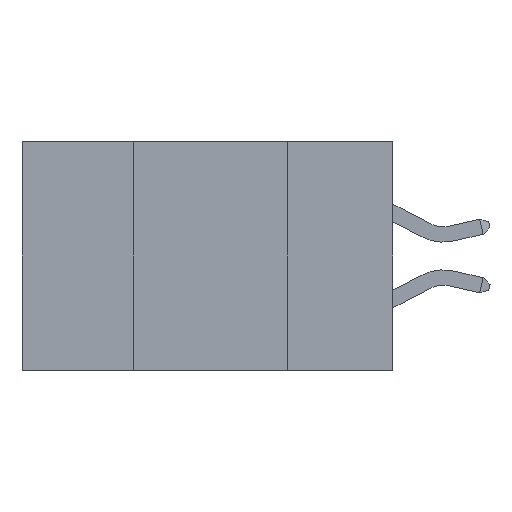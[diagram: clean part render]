
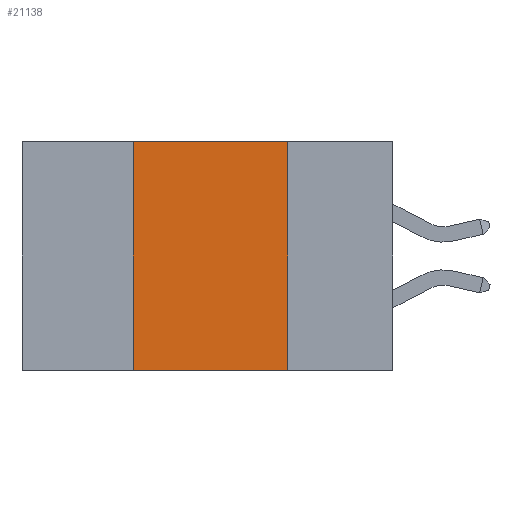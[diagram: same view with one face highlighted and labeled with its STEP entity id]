
A CAD part, left-side view. The second image highlights one B-rep face of the part: STEP entity #21138.
In plain terms, the highlighted planar face has unit normal (-1, 0, 0).
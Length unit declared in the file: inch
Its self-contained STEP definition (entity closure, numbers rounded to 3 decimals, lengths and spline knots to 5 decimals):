
#1626 = VERTEX_POINT ( 'NONE', #39096 ) ;
#4777 = AXIS2_PLACEMENT_3D ( 'NONE', #39621, #43118, #22553 ) ;
#5288 = DIRECTION ( 'NONE',  ( 0., 0., -1. ) ) ;
#8148 = LINE ( 'NONE', #11508, #25239 ) ;
#11380 = VECTOR ( 'NONE', #37002, 39.37008 ) ;
#11508 = CARTESIAN_POINT ( 'NONE',  ( 0., 0.6, 0. ) ) ;
#12672 = EDGE_CURVE ( 'NONE', #1626, #31656, #37757, .T. ) ;
#14504 = EDGE_CURVE ( 'NONE', #21414, #1626, #8148, .T. ) ;
#14821 = ORIENTED_EDGE ( 'NONE', *, *, #43545, .T. ) ;
#14949 = DIRECTION ( 'NONE',  ( 0., -1., 0. ) ) ;
#15928 = ORIENTED_EDGE ( 'NONE', *, *, #14504, .F. ) ;
#19158 = ORIENTED_EDGE ( 'NONE', *, *, #12672, .F. ) ;
#19921 = CARTESIAN_POINT ( 'NONE',  ( 0., 0.6, -0.37 ) ) ;
#20589 = VECTOR ( 'NONE', #5288, 39.37008 ) ;
#21138 = ADVANCED_FACE ( 'NONE', ( #31161 ), #32733, .F. ) ;
#21414 = VERTEX_POINT ( 'NONE', #23954 ) ;
#21919 = CARTESIAN_POINT ( 'NONE',  ( 0., 0.17, -0.37 ) ) ;
#22553 = DIRECTION ( 'NONE',  ( 0., 0., -1. ) ) ;
#23954 = CARTESIAN_POINT ( 'NONE',  ( 0., 0.42, 0. ) ) ;
#24689 = VECTOR ( 'NONE', #28709, 39.37008 ) ;
#25239 = VECTOR ( 'NONE', #14949, 39.37008 ) ;
#28709 = DIRECTION ( 'NONE',  ( 0., 0., 1. ) ) ;
#29187 = CARTESIAN_POINT ( 'NONE',  ( 0., 0.17, 0. ) ) ;
#29583 = LINE ( 'NONE', #19921, #11380 ) ;
#30359 = ORIENTED_EDGE ( 'NONE', *, *, #32325, .F. ) ;
#31161 = FACE_OUTER_BOUND ( 'NONE', #39514, .T. ) ;
#31656 = VERTEX_POINT ( 'NONE', #21919 ) ;
#32325 = EDGE_CURVE ( 'NONE', #36967, #21414, #42944, .T. ) ;
#32733 = PLANE ( 'NONE',  #4777 ) ;
#35500 = CARTESIAN_POINT ( 'NONE',  ( 0., 0.42, 0. ) ) ;
#36967 = VERTEX_POINT ( 'NONE', #38968 ) ;
#37002 = DIRECTION ( 'NONE',  ( 0., -1., 0. ) ) ;
#37757 = LINE ( 'NONE', #29187, #20589 ) ;
#38968 = CARTESIAN_POINT ( 'NONE',  ( 0., 0.42, -0.37 ) ) ;
#39096 = CARTESIAN_POINT ( 'NONE',  ( 0., 0.17, 0. ) ) ;
#39514 = EDGE_LOOP ( 'NONE', ( #19158, #15928, #30359, #14821 ) ) ;
#39621 = CARTESIAN_POINT ( 'NONE',  ( 0., 0.6, 0. ) ) ;
#42944 = LINE ( 'NONE', #35500, #24689 ) ;
#43118 = DIRECTION ( 'NONE',  ( 1., 0., 0. ) ) ;
#43545 = EDGE_CURVE ( 'NONE', #36967, #31656, #29583, .T. ) ;
